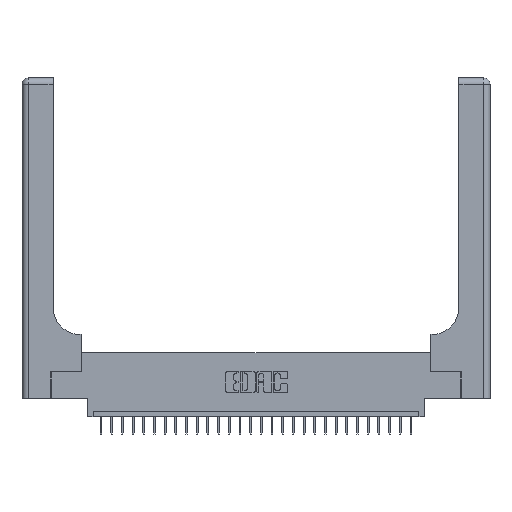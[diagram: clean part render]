
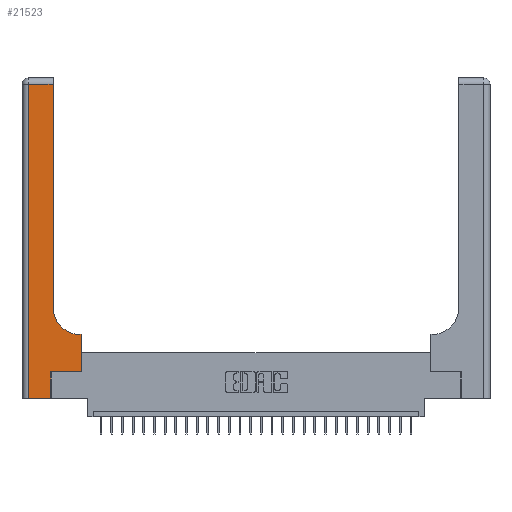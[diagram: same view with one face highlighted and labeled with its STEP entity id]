
A CAD part, top view. The second image highlights one B-rep face of the part: STEP entity #21523.
In plain terms, the highlighted planar face has unit normal (0, 0, 1).
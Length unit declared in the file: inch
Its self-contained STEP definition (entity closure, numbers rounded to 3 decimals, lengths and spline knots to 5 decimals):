
#1156 = CARTESIAN_POINT ( 'NONE',  ( 0.269, 0., 0.37 ) ) ;
#1258 = AXIS2_PLACEMENT_3D ( 'NONE', #16528, #11939, #2747 ) ;
#2547 = CARTESIAN_POINT ( 'NONE',  ( 0., 3., 0.37 ) ) ;
#2747 = DIRECTION ( 'NONE',  ( 1., 0., 0. ) ) ;
#2758 = DIRECTION ( 'NONE',  ( 0., 1., 0. ) ) ;
#3185 = CARTESIAN_POINT ( 'NONE',  ( 0.2915, 2.94, 0.37 ) ) ;
#3368 = EDGE_CURVE ( 'NONE', #28478, #19936, #16420, .T. ) ;
#3980 = CARTESIAN_POINT ( 'NONE',  ( 0.269, 0., 0.37 ) ) ;
#4127 = ORIENTED_EDGE ( 'NONE', *, *, #10340, .T. ) ;
#4816 = VECTOR ( 'NONE', #2758, 39.37008 ) ;
#4924 = DIRECTION ( 'NONE',  ( 0., 0., -1. ) ) ;
#4954 = VECTOR ( 'NONE', #27402, 39.37008 ) ;
#5005 = ORIENTED_EDGE ( 'NONE', *, *, #14940, .T. ) ;
#5426 = DIRECTION ( 'NONE',  ( -1., 0., 0. ) ) ;
#5660 = ORIENTED_EDGE ( 'NONE', *, *, #25013, .T. ) ;
#6640 = LINE ( 'NONE', #25212, #4816 ) ;
#6789 = FACE_OUTER_BOUND ( 'NONE', #7542, .T. ) ;
#6993 = DIRECTION ( 'NONE',  ( 1., 0., 0. ) ) ;
#7014 = CARTESIAN_POINT ( 'NONE',  ( 0.2915, 3., 0.37 ) ) ;
#7303 = LINE ( 'NONE', #23559, #21607 ) ;
#7542 = EDGE_LOOP ( 'NONE', ( #9175, #5660, #16841, #5005, #12847, #18068, #13301, #4127, #27911 ) ) ;
#7715 = DIRECTION ( 'NONE',  ( 0., 1., 0. ) ) ;
#7718 = DIRECTION ( 'NONE',  ( -1., 0., 0. ) ) ;
#9125 = VECTOR ( 'NONE', #6993, 39.37008 ) ;
#9172 = EDGE_CURVE ( 'NONE', #13186, #24856, #20719, .T. ) ;
#9175 = ORIENTED_EDGE ( 'NONE', *, *, #21763, .T. ) ;
#10340 = EDGE_CURVE ( 'NONE', #23556, #11469, #7303, .T. ) ;
#10373 = VECTOR ( 'NONE', #5426, 39.37008 ) ;
#11183 = CARTESIAN_POINT ( 'NONE',  ( 0.269, 0.25, 0.37 ) ) ;
#11469 = VERTEX_POINT ( 'NONE', #13175 ) ;
#11939 = DIRECTION ( 'NONE',  ( 0., 0., -1. ) ) ;
#12119 = CARTESIAN_POINT ( 'NONE',  ( 0.5585, 0.25, 0.37 ) ) ;
#12510 = CARTESIAN_POINT ( 'NONE',  ( 0.2915, 0.85, 0.37 ) ) ;
#12847 = ORIENTED_EDGE ( 'NONE', *, *, #3368, .T. ) ;
#12900 = VERTEX_POINT ( 'NONE', #12510 ) ;
#13175 = CARTESIAN_POINT ( 'NONE',  ( 0.5415, 0.6, 0.37 ) ) ;
#13186 = VERTEX_POINT ( 'NONE', #22165 ) ;
#13301 = ORIENTED_EDGE ( 'NONE', *, *, #26979, .T. ) ;
#14940 = EDGE_CURVE ( 'NONE', #24856, #28478, #28088, .T. ) ;
#15383 = EDGE_CURVE ( 'NONE', #19936, #28715, #27337, .T. ) ;
#15451 = CARTESIAN_POINT ( 'NONE',  ( 0.5585, 0.6, 0.37 ) ) ;
#16420 = LINE ( 'NONE', #1156, #27865 ) ;
#16512 = CARTESIAN_POINT ( 'NONE',  ( 0., 0., 0.37 ) ) ;
#16528 = CARTESIAN_POINT ( 'NONE',  ( 0.5415, 0.85, 0.37 ) ) ;
#16841 = ORIENTED_EDGE ( 'NONE', *, *, #9172, .T. ) ;
#17104 = CARTESIAN_POINT ( 'NONE',  ( 0.06, 3., 0.37 ) ) ;
#18068 = ORIENTED_EDGE ( 'NONE', *, *, #15383, .T. ) ;
#18781 = CARTESIAN_POINT ( 'NONE',  ( 0.269, 0.25, 0.37 ) ) ;
#19302 = DIRECTION ( 'NONE',  ( 0., -1., 0. ) ) ;
#19632 = LINE ( 'NONE', #7014, #4954 ) ;
#19936 = VERTEX_POINT ( 'NONE', #11183 ) ;
#20626 = CARTESIAN_POINT ( 'NONE',  ( 0.06, 0., 0.37 ) ) ;
#20719 = LINE ( 'NONE', #17104, #21396 ) ;
#20914 = PLANE ( 'NONE',  #23333 ) ;
#21396 = VECTOR ( 'NONE', #19302, 39.37008 ) ;
#21397 = LINE ( 'NONE', #23598, #10373 ) ;
#21523 = ADVANCED_FACE ( 'NONE', ( #6789 ), #20914, .F. ) ;
#21607 = VECTOR ( 'NONE', #7718, 39.37008 ) ;
#21763 = EDGE_CURVE ( 'NONE', #12900, #22644, #19632, .T. ) ;
#22165 = CARTESIAN_POINT ( 'NONE',  ( 0.06, 2.94, 0.37 ) ) ;
#22644 = VERTEX_POINT ( 'NONE', #3185 ) ;
#23333 = AXIS2_PLACEMENT_3D ( 'NONE', #2547, #4924, #25494 ) ;
#23385 = DIRECTION ( 'NONE',  ( 1., 0., 0. ) ) ;
#23556 = VERTEX_POINT ( 'NONE', #15451 ) ;
#23559 = CARTESIAN_POINT ( 'NONE',  ( 0.2915, 0.6, 0.37 ) ) ;
#23598 = CARTESIAN_POINT ( 'NONE',  ( 0., 2.94, 0.37 ) ) ;
#24839 = EDGE_CURVE ( 'NONE', #11469, #12900, #24990, .T. ) ;
#24856 = VERTEX_POINT ( 'NONE', #20626 ) ;
#24990 = CIRCLE ( 'NONE', #1258, 0.25 ) ;
#25013 = EDGE_CURVE ( 'NONE', #22644, #13186, #21397, .T. ) ;
#25201 = VECTOR ( 'NONE', #23385, 39.37008 ) ;
#25212 = CARTESIAN_POINT ( 'NONE',  ( 0.5585, 0.25, 0.37 ) ) ;
#25494 = DIRECTION ( 'NONE',  ( -1., 0., 0. ) ) ;
#26979 = EDGE_CURVE ( 'NONE', #28715, #23556, #6640, .T. ) ;
#27337 = LINE ( 'NONE', #18781, #9125 ) ;
#27402 = DIRECTION ( 'NONE',  ( 0., 1., 0. ) ) ;
#27865 = VECTOR ( 'NONE', #7715, 39.37008 ) ;
#27911 = ORIENTED_EDGE ( 'NONE', *, *, #24839, .T. ) ;
#28088 = LINE ( 'NONE', #16512, #25201 ) ;
#28478 = VERTEX_POINT ( 'NONE', #3980 ) ;
#28715 = VERTEX_POINT ( 'NONE', #12119 ) ;
